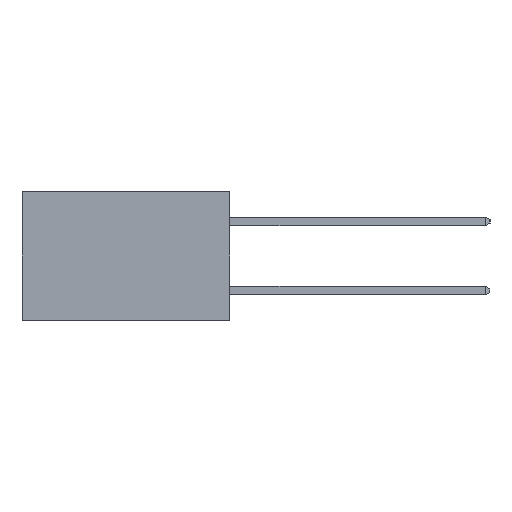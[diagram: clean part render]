
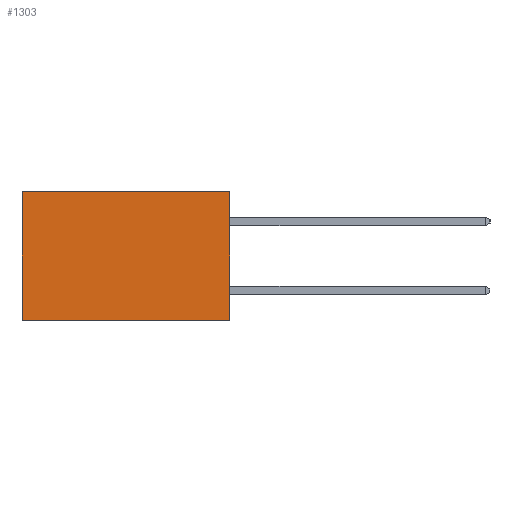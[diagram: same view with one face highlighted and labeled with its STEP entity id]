
A CAD part, left-side view. The second image highlights one B-rep face of the part: STEP entity #1303.
In plain terms, the highlighted planar face has unit normal (-1, 0, 0).
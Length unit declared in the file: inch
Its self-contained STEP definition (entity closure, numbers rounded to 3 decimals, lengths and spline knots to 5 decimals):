
#721 = VERTEX_POINT ( 'NONE', #4935 ) ;
#738 = CARTESIAN_POINT ( 'NONE',  ( 0.298, 0., -0.37 ) ) ;
#740 = VECTOR ( 'NONE', #9938, 39.37008 ) ;
#870 = VERTEX_POINT ( 'NONE', #4467 ) ;
#1303 = ADVANCED_FACE ( 'NONE', ( #5415 ), #8318, .F. ) ;
#1359 = LINE ( 'NONE', #8388, #9895 ) ;
#2671 = ORIENTED_EDGE ( 'NONE', *, *, #5474, .T. ) ;
#2806 = CARTESIAN_POINT ( 'NONE',  ( 0.298, 0.6, 0. ) ) ;
#3460 = EDGE_CURVE ( 'NONE', #721, #870, #10039, .T. ) ;
#3826 = LINE ( 'NONE', #7870, #7756 ) ;
#3871 = VECTOR ( 'NONE', #9525, 39.37008 ) ;
#3927 = CARTESIAN_POINT ( 'NONE',  ( 0.298, 0., 0. ) ) ;
#3980 = LINE ( 'NONE', #2806, #740 ) ;
#4072 = CARTESIAN_POINT ( 'NONE',  ( 0.298, 0., 0. ) ) ;
#4074 = ORIENTED_EDGE ( 'NONE', *, *, #7498, .F. ) ;
#4467 = CARTESIAN_POINT ( 'NONE',  ( 0.298, 0.6, 0. ) ) ;
#4841 = ORIENTED_EDGE ( 'NONE', *, *, #3460, .T. ) ;
#4935 = CARTESIAN_POINT ( 'NONE',  ( 0.298, 0., 0. ) ) ;
#5415 = FACE_OUTER_BOUND ( 'NONE', #7083, .T. ) ;
#5474 = EDGE_CURVE ( 'NONE', #870, #9036, #3980, .T. ) ;
#6052 = DIRECTION ( 'NONE',  ( 0., 1., 0. ) ) ;
#6062 = ORIENTED_EDGE ( 'NONE', *, *, #7249, .F. ) ;
#6591 = DIRECTION ( 'NONE',  ( 0., 0., -1. ) ) ;
#7083 = EDGE_LOOP ( 'NONE', ( #2671, #6062, #4074, #4841 ) ) ;
#7249 = EDGE_CURVE ( 'NONE', #10300, #9036, #1359, .T. ) ;
#7498 = EDGE_CURVE ( 'NONE', #721, #10300, #3826, .T. ) ;
#7500 = DIRECTION ( 'NONE',  ( 1., 0., 0. ) ) ;
#7696 = AXIS2_PLACEMENT_3D ( 'NONE', #3927, #7500, #6591 ) ;
#7756 = VECTOR ( 'NONE', #8617, 39.37008 ) ;
#7870 = CARTESIAN_POINT ( 'NONE',  ( 0.298, 0., 0. ) ) ;
#8281 = CARTESIAN_POINT ( 'NONE',  ( 0.298, 0.6, -0.37 ) ) ;
#8318 = PLANE ( 'NONE',  #7696 ) ;
#8388 = CARTESIAN_POINT ( 'NONE',  ( 0.298, 0., -0.37 ) ) ;
#8617 = DIRECTION ( 'NONE',  ( 0., 0., -1. ) ) ;
#9036 = VERTEX_POINT ( 'NONE', #8281 ) ;
#9525 = DIRECTION ( 'NONE',  ( 0., 1., 0. ) ) ;
#9895 = VECTOR ( 'NONE', #6052, 39.37008 ) ;
#9938 = DIRECTION ( 'NONE',  ( 0., 0., -1. ) ) ;
#10039 = LINE ( 'NONE', #4072, #3871 ) ;
#10300 = VERTEX_POINT ( 'NONE', #738 ) ;
